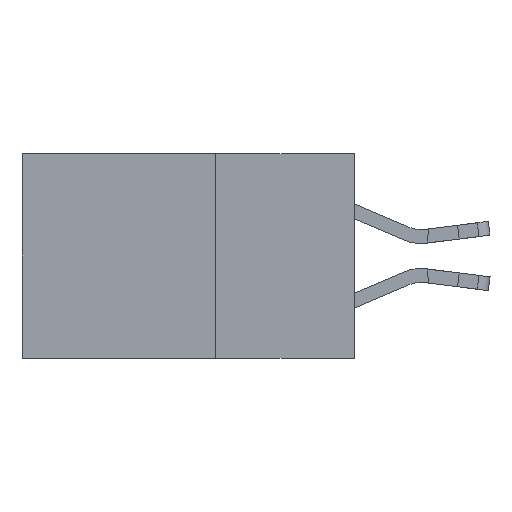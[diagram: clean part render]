
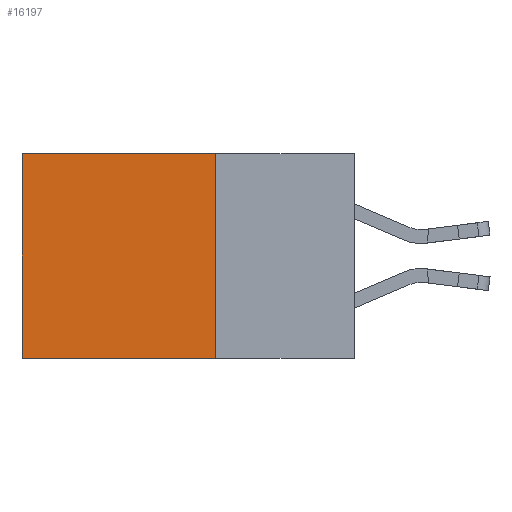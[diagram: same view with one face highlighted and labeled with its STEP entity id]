
A CAD part, left-side view. The second image highlights one B-rep face of the part: STEP entity #16197.
In plain terms, the highlighted planar face has unit normal (-1, 0, 0).
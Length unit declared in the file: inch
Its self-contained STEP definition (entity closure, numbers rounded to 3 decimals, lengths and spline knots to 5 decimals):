
#626 = CARTESIAN_POINT ( 'NONE',  ( 0.298, 0.25, 0. ) ) ;
#906 = LINE ( 'NONE', #15573, #13842 ) ;
#1985 = LINE ( 'NONE', #7718, #2576 ) ;
#2335 = VERTEX_POINT ( 'NONE', #4318 ) ;
#2576 = VECTOR ( 'NONE', #10300, 39.37008 ) ;
#2613 = DIRECTION ( 'NONE',  ( 0., 1., 0. ) ) ;
#3373 = PLANE ( 'NONE',  #9568 ) ;
#3584 = VERTEX_POINT ( 'NONE', #9502 ) ;
#4318 = CARTESIAN_POINT ( 'NONE',  ( 0.298, 0.6, 0. ) ) ;
#5103 = VERTEX_POINT ( 'NONE', #15615 ) ;
#6189 = CARTESIAN_POINT ( 'NONE',  ( 0.298, 0.25, -0.37 ) ) ;
#7203 = ORIENTED_EDGE ( 'NONE', *, *, #10556, .T. ) ;
#7237 = FACE_OUTER_BOUND ( 'NONE', #8724, .T. ) ;
#7420 = LINE ( 'NONE', #8878, #14496 ) ;
#7718 = CARTESIAN_POINT ( 'NONE',  ( 0.298, 0.25, 0. ) ) ;
#7916 = EDGE_CURVE ( 'NONE', #3584, #2335, #1985, .T. ) ;
#8702 = CARTESIAN_POINT ( 'NONE',  ( 0.298, 0.6, 0. ) ) ;
#8724 = EDGE_LOOP ( 'NONE', ( #7203, #15068, #14304, #10979 ) ) ;
#8878 = CARTESIAN_POINT ( 'NONE',  ( 0.298, 0.25, -0.37 ) ) ;
#9465 = VECTOR ( 'NONE', #11234, 39.37008 ) ;
#9502 = CARTESIAN_POINT ( 'NONE',  ( 0.298, 0.25, 0. ) ) ;
#9568 = AXIS2_PLACEMENT_3D ( 'NONE', #626, #12358, #16125 ) ;
#10298 = DIRECTION ( 'NONE',  ( 0., 0., -1. ) ) ;
#10300 = DIRECTION ( 'NONE',  ( 0., 1., 0. ) ) ;
#10556 = EDGE_CURVE ( 'NONE', #2335, #5103, #12072, .T. ) ;
#10916 = VERTEX_POINT ( 'NONE', #6189 ) ;
#10979 = ORIENTED_EDGE ( 'NONE', *, *, #7916, .T. ) ;
#11234 = DIRECTION ( 'NONE',  ( 0., 0., -1. ) ) ;
#11770 = EDGE_CURVE ( 'NONE', #3584, #10916, #906, .T. ) ;
#12072 = LINE ( 'NONE', #8702, #9465 ) ;
#12358 = DIRECTION ( 'NONE',  ( 1., 0., 0. ) ) ;
#13842 = VECTOR ( 'NONE', #10298, 39.37008 ) ;
#14304 = ORIENTED_EDGE ( 'NONE', *, *, #11770, .F. ) ;
#14496 = VECTOR ( 'NONE', #2613, 39.37008 ) ;
#15068 = ORIENTED_EDGE ( 'NONE', *, *, #16424, .F. ) ;
#15573 = CARTESIAN_POINT ( 'NONE',  ( 0.298, 0.25, 0. ) ) ;
#15615 = CARTESIAN_POINT ( 'NONE',  ( 0.298, 0.6, -0.37 ) ) ;
#16125 = DIRECTION ( 'NONE',  ( 0., 0., -1. ) ) ;
#16197 = ADVANCED_FACE ( 'NONE', ( #7237 ), #3373, .F. ) ;
#16424 = EDGE_CURVE ( 'NONE', #10916, #5103, #7420, .T. ) ;
